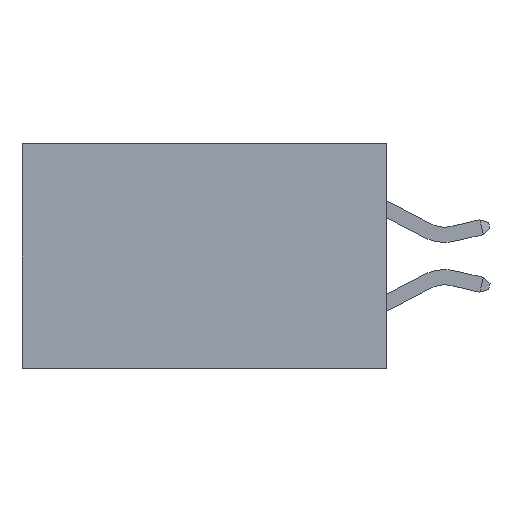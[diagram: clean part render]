
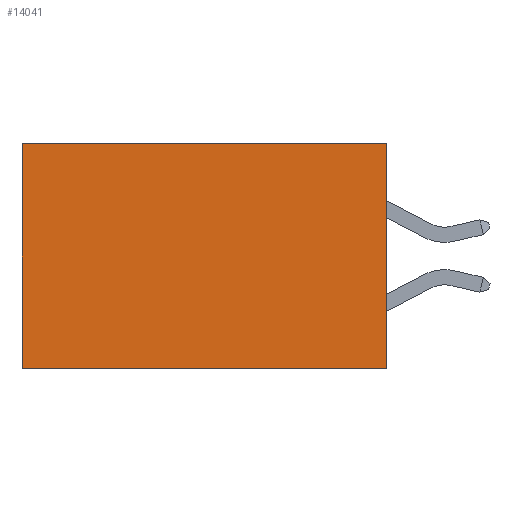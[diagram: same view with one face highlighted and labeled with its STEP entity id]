
A CAD part, left-side view. The second image highlights one B-rep face of the part: STEP entity #14041.
In plain terms, the highlighted planar face has unit normal (-1, 0, 0).
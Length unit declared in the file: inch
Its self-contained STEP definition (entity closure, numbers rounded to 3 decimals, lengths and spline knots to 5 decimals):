
#363 = FACE_OUTER_BOUND ( 'NONE', #1266, .T. ) ;
#441 = VECTOR ( 'NONE', #10986, 39.37008 ) ;
#1266 = EDGE_LOOP ( 'NONE', ( #6205, #12214, #12587, #5023 ) ) ;
#1373 = DIRECTION ( 'NONE',  ( 0., 0., -1. ) ) ;
#1379 = DIRECTION ( 'NONE',  ( 1., 0., 0. ) ) ;
#1396 = CARTESIAN_POINT ( 'NONE',  ( 0.2615, 0., -0.37 ) ) ;
#1551 = PLANE ( 'NONE',  #7382 ) ;
#3063 = CARTESIAN_POINT ( 'NONE',  ( 0.2615, 0., 0. ) ) ;
#3388 = LINE ( 'NONE', #12857, #441 ) ;
#4313 = CARTESIAN_POINT ( 'NONE',  ( 0.2615, 0., -0.37 ) ) ;
#4781 = DIRECTION ( 'NONE',  ( 0., 1., 0. ) ) ;
#4828 = CARTESIAN_POINT ( 'NONE',  ( 0.2615, 0., -0.37 ) ) ;
#5023 = ORIENTED_EDGE ( 'NONE', *, *, #8311, .T. ) ;
#5215 = VECTOR ( 'NONE', #4781, 39.37008 ) ;
#5623 = EDGE_CURVE ( 'NONE', #8685, #11958, #13951, .T. ) ;
#6205 = ORIENTED_EDGE ( 'NONE', *, *, #5623, .T. ) ;
#6722 = EDGE_CURVE ( 'NONE', #6756, #11958, #14782, .T. ) ;
#6756 = VERTEX_POINT ( 'NONE', #4313 ) ;
#7382 = AXIS2_PLACEMENT_3D ( 'NONE', #1396, #1379, #1373 ) ;
#8311 = EDGE_CURVE ( 'NONE', #9382, #8685, #8320, .T. ) ;
#8320 = LINE ( 'NONE', #14119, #13538 ) ;
#8353 = EDGE_CURVE ( 'NONE', #9382, #6756, #3388, .T. ) ;
#8685 = VERTEX_POINT ( 'NONE', #10876 ) ;
#8874 = CARTESIAN_POINT ( 'NONE',  ( 0.2615, 0.6, -0.37 ) ) ;
#9382 = VERTEX_POINT ( 'NONE', #3063 ) ;
#10210 = DIRECTION ( 'NONE',  ( 0., 0., -1. ) ) ;
#10489 = VECTOR ( 'NONE', #10210, 39.37008 ) ;
#10876 = CARTESIAN_POINT ( 'NONE',  ( 0.2615, 0.6, 0. ) ) ;
#10986 = DIRECTION ( 'NONE',  ( 0., 0., -1. ) ) ;
#11143 = CARTESIAN_POINT ( 'NONE',  ( 0.2615, 0.6, -0.37 ) ) ;
#11421 = DIRECTION ( 'NONE',  ( 0., 1., 0. ) ) ;
#11958 = VERTEX_POINT ( 'NONE', #11143 ) ;
#12214 = ORIENTED_EDGE ( 'NONE', *, *, #6722, .F. ) ;
#12587 = ORIENTED_EDGE ( 'NONE', *, *, #8353, .F. ) ;
#12857 = CARTESIAN_POINT ( 'NONE',  ( 0.2615, 0., -0.37 ) ) ;
#13538 = VECTOR ( 'NONE', #11421, 39.37008 ) ;
#13951 = LINE ( 'NONE', #8874, #10489 ) ;
#14041 = ADVANCED_FACE ( 'NONE', ( #363 ), #1551, .F. ) ;
#14119 = CARTESIAN_POINT ( 'NONE',  ( 0.2615, 0., 0. ) ) ;
#14782 = LINE ( 'NONE', #4828, #5215 ) ;
